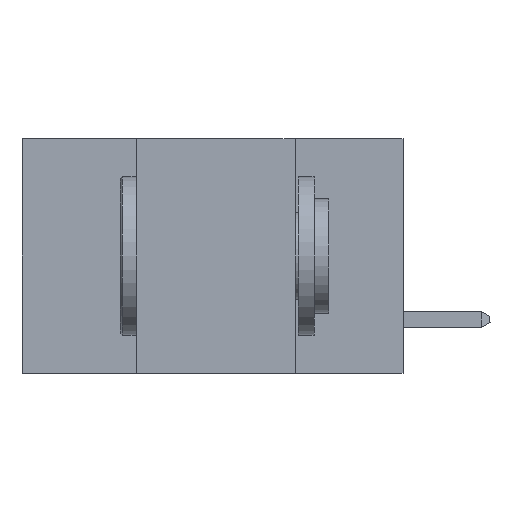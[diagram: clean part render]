
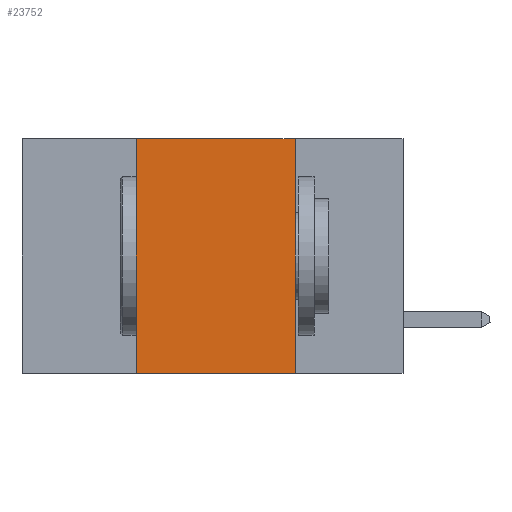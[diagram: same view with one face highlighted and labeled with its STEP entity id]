
A CAD part, left-side view. The second image highlights one B-rep face of the part: STEP entity #23752.
In plain terms, the highlighted planar face has unit normal (-1, 0, 0).
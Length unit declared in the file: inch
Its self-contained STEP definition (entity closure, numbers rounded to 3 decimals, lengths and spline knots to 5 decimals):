
#1019 = LINE ( 'NONE', #19863, #21148 ) ;
#1718 = ORIENTED_EDGE ( 'NONE', *, *, #21873, .F. ) ;
#2582 = VERTEX_POINT ( 'NONE', #12791 ) ;
#4689 = VERTEX_POINT ( 'NONE', #22083 ) ;
#4814 = VERTEX_POINT ( 'NONE', #22427 ) ;
#6771 = EDGE_CURVE ( 'NONE', #4814, #2582, #16348, .T. ) ;
#7400 = AXIS2_PLACEMENT_3D ( 'NONE', #9320, #26272, #18031 ) ;
#8595 = VERTEX_POINT ( 'NONE', #25457 ) ;
#9229 = VECTOR ( 'NONE', #15190, 39.37008 ) ;
#9320 = CARTESIAN_POINT ( 'NONE',  ( 0., 0.6, 0. ) ) ;
#11394 = LINE ( 'NONE', #26866, #22081 ) ;
#12186 = LINE ( 'NONE', #14618, #21930 ) ;
#12791 = CARTESIAN_POINT ( 'NONE',  ( 0., 0.17, -0.37 ) ) ;
#13109 = CARTESIAN_POINT ( 'NONE',  ( 0., 0.17, 0. ) ) ;
#14618 = CARTESIAN_POINT ( 'NONE',  ( 0., 0.6, 0. ) ) ;
#14877 = DIRECTION ( 'NONE',  ( 0., -1., 0. ) ) ;
#15190 = DIRECTION ( 'NONE',  ( 0., 0., -1. ) ) ;
#16276 = ORIENTED_EDGE ( 'NONE', *, *, #18006, .T. ) ;
#16348 = LINE ( 'NONE', #13109, #9229 ) ;
#17012 = DIRECTION ( 'NONE',  ( 0., 0., 1. ) ) ;
#17275 = ORIENTED_EDGE ( 'NONE', *, *, #6771, .F. ) ;
#18006 = EDGE_CURVE ( 'NONE', #4689, #2582, #1019, .T. ) ;
#18031 = DIRECTION ( 'NONE',  ( 0., 0., -1. ) ) ;
#18514 = EDGE_CURVE ( 'NONE', #4689, #8595, #11394, .T. ) ;
#19849 = EDGE_LOOP ( 'NONE', ( #17275, #1718, #20393, #16276 ) ) ;
#19863 = CARTESIAN_POINT ( 'NONE',  ( 0., 0.6, -0.37 ) ) ;
#20393 = ORIENTED_EDGE ( 'NONE', *, *, #18514, .F. ) ;
#21148 = VECTOR ( 'NONE', #21936, 39.37008 ) ;
#21873 = EDGE_CURVE ( 'NONE', #8595, #4814, #12186, .T. ) ;
#21930 = VECTOR ( 'NONE', #14877, 39.37008 ) ;
#21936 = DIRECTION ( 'NONE',  ( 0., -1., 0. ) ) ;
#22081 = VECTOR ( 'NONE', #17012, 39.37008 ) ;
#22083 = CARTESIAN_POINT ( 'NONE',  ( 0., 0.42, -0.37 ) ) ;
#22140 = FACE_OUTER_BOUND ( 'NONE', #19849, .T. ) ;
#22427 = CARTESIAN_POINT ( 'NONE',  ( 0., 0.17, 0. ) ) ;
#23752 = ADVANCED_FACE ( 'NONE', ( #22140 ), #24414, .F. ) ;
#24414 = PLANE ( 'NONE',  #7400 ) ;
#25457 = CARTESIAN_POINT ( 'NONE',  ( 0., 0.42, 0. ) ) ;
#26272 = DIRECTION ( 'NONE',  ( 1., 0., 0. ) ) ;
#26866 = CARTESIAN_POINT ( 'NONE',  ( 0., 0.42, 0. ) ) ;
